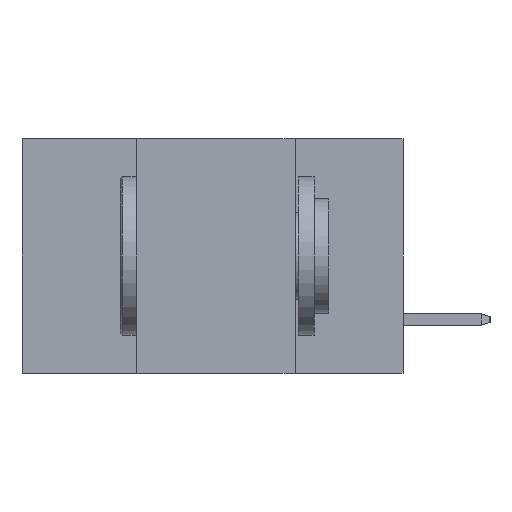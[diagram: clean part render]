
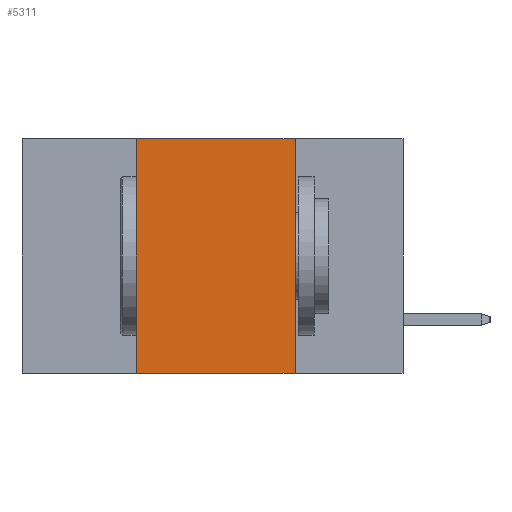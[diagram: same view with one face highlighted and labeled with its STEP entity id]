
A CAD part, left-side view. The second image highlights one B-rep face of the part: STEP entity #5311.
In plain terms, the highlighted planar face has unit normal (-1, 0, 0).
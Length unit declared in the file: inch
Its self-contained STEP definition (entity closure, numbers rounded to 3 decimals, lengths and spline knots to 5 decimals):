
#61 = VECTOR ( 'NONE', #6016, 39.37008 ) ;
#243 = VERTEX_POINT ( 'NONE', #16365 ) ;
#475 = ORIENTED_EDGE ( 'NONE', *, *, #10314, .T. ) ;
#519 = AXIS2_PLACEMENT_3D ( 'NONE', #9828, #16369, #8704 ) ;
#1498 = ORIENTED_EDGE ( 'NONE', *, *, #16962, .F. ) ;
#1869 = CARTESIAN_POINT ( 'NONE',  ( 0., 0.42, -0.37 ) ) ;
#1913 = EDGE_CURVE ( 'NONE', #15653, #7628, #10154, .T. ) ;
#1945 = DIRECTION ( 'NONE',  ( 0., 0., 1. ) ) ;
#2339 = EDGE_CURVE ( 'NONE', #15266, #15653, #9782, .T. ) ;
#3599 = EDGE_LOOP ( 'NONE', ( #1498, #4983, #7402, #475 ) ) ;
#4650 = LINE ( 'NONE', #7221, #61 ) ;
#4983 = ORIENTED_EDGE ( 'NONE', *, *, #1913, .F. ) ;
#5311 = ADVANCED_FACE ( 'NONE', ( #6049 ), #11304, .F. ) ;
#6016 = DIRECTION ( 'NONE',  ( 0., -1., 0. ) ) ;
#6049 = FACE_OUTER_BOUND ( 'NONE', #3599, .T. ) ;
#7221 = CARTESIAN_POINT ( 'NONE',  ( 0., 0.6, -0.37 ) ) ;
#7398 = CARTESIAN_POINT ( 'NONE',  ( 0., 0.6, 0. ) ) ;
#7402 = ORIENTED_EDGE ( 'NONE', *, *, #2339, .F. ) ;
#7628 = VERTEX_POINT ( 'NONE', #12022 ) ;
#8383 = DIRECTION ( 'NONE',  ( 0., 0., -1. ) ) ;
#8704 = DIRECTION ( 'NONE',  ( 0., 0., -1. ) ) ;
#9782 = LINE ( 'NONE', #15119, #10911 ) ;
#9828 = CARTESIAN_POINT ( 'NONE',  ( 0., 0.6, 0. ) ) ;
#9900 = CARTESIAN_POINT ( 'NONE',  ( 0., 0.42, 0. ) ) ;
#9925 = LINE ( 'NONE', #13709, #13218 ) ;
#10154 = LINE ( 'NONE', #7398, #14291 ) ;
#10314 = EDGE_CURVE ( 'NONE', #15266, #243, #4650, .T. ) ;
#10911 = VECTOR ( 'NONE', #1945, 39.37008 ) ;
#11280 = DIRECTION ( 'NONE',  ( 0., -1., 0. ) ) ;
#11304 = PLANE ( 'NONE',  #519 ) ;
#12022 = CARTESIAN_POINT ( 'NONE',  ( 0., 0.17, 0. ) ) ;
#13218 = VECTOR ( 'NONE', #8383, 39.37008 ) ;
#13709 = CARTESIAN_POINT ( 'NONE',  ( 0., 0.17, 0. ) ) ;
#14291 = VECTOR ( 'NONE', #11280, 39.37008 ) ;
#15119 = CARTESIAN_POINT ( 'NONE',  ( 0., 0.42, 0. ) ) ;
#15266 = VERTEX_POINT ( 'NONE', #1869 ) ;
#15653 = VERTEX_POINT ( 'NONE', #9900 ) ;
#16365 = CARTESIAN_POINT ( 'NONE',  ( 0., 0.17, -0.37 ) ) ;
#16369 = DIRECTION ( 'NONE',  ( 1., 0., 0. ) ) ;
#16962 = EDGE_CURVE ( 'NONE', #7628, #243, #9925, .T. ) ;
